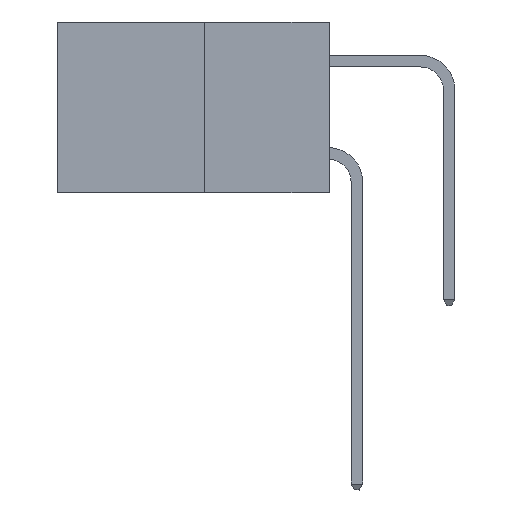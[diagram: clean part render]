
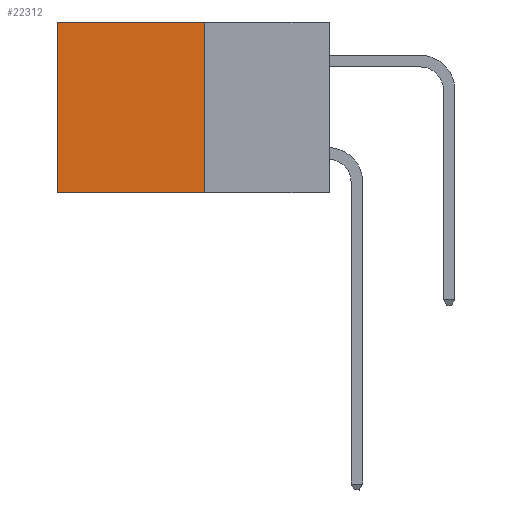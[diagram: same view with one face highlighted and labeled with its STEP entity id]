
A CAD part, left-side view. The second image highlights one B-rep face of the part: STEP entity #22312.
In plain terms, the highlighted planar face has unit normal (-1, 0, 0).
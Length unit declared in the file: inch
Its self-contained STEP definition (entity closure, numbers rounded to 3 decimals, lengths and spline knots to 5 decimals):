
#1403 = VECTOR ( 'NONE', #1879, 39.37008 ) ;
#1879 = DIRECTION ( 'NONE',  ( 0., 0., -1. ) ) ;
#2304 = CARTESIAN_POINT ( 'NONE',  ( 0.277, 0.59, -0.37 ) ) ;
#2451 = PLANE ( 'NONE',  #21595 ) ;
#4678 = ORIENTED_EDGE ( 'NONE', *, *, #18040, .F. ) ;
#8793 = ORIENTED_EDGE ( 'NONE', *, *, #16566, .F. ) ;
#9172 = CARTESIAN_POINT ( 'NONE',  ( 0.277, 0.27, -0.37 ) ) ;
#9615 = CARTESIAN_POINT ( 'NONE',  ( 0.277, 0.59, 0. ) ) ;
#10212 = VECTOR ( 'NONE', #12533, 39.37008 ) ;
#10831 = CARTESIAN_POINT ( 'NONE',  ( 0.277, 0.27, 0. ) ) ;
#10929 = VERTEX_POINT ( 'NONE', #10831 ) ;
#11396 = DIRECTION ( 'NONE',  ( 0., 0., -1. ) ) ;
#11612 = CARTESIAN_POINT ( 'NONE',  ( 0.277, 0.27, 0. ) ) ;
#11629 = LINE ( 'NONE', #21446, #10212 ) ;
#12533 = DIRECTION ( 'NONE',  ( 0., 1., 0. ) ) ;
#13137 = EDGE_CURVE ( 'NONE', #27296, #15445, #18124, .T. ) ;
#14676 = LINE ( 'NONE', #28496, #1403 ) ;
#15445 = VERTEX_POINT ( 'NONE', #2304 ) ;
#16566 = EDGE_CURVE ( 'NONE', #26795, #15445, #11629, .T. ) ;
#16731 = VECTOR ( 'NONE', #18975, 39.37008 ) ;
#16745 = VECTOR ( 'NONE', #20580, 39.37008 ) ;
#17876 = CARTESIAN_POINT ( 'NONE',  ( 0.277, 0.27, -0.37 ) ) ;
#18040 = EDGE_CURVE ( 'NONE', #10929, #26795, #14676, .T. ) ;
#18124 = LINE ( 'NONE', #18866, #16731 ) ;
#18289 = EDGE_CURVE ( 'NONE', #10929, #27296, #22664, .T. ) ;
#18866 = CARTESIAN_POINT ( 'NONE',  ( 0.277, 0.59, -0.37 ) ) ;
#18975 = DIRECTION ( 'NONE',  ( 0., 0., -1. ) ) ;
#20580 = DIRECTION ( 'NONE',  ( 0., 1., 0. ) ) ;
#21446 = CARTESIAN_POINT ( 'NONE',  ( 0.277, 0.27, -0.37 ) ) ;
#21567 = EDGE_LOOP ( 'NONE', ( #21814, #8793, #4678, #23461 ) ) ;
#21595 = AXIS2_PLACEMENT_3D ( 'NONE', #9172, #24748, #11396 ) ;
#21814 = ORIENTED_EDGE ( 'NONE', *, *, #13137, .T. ) ;
#22312 = ADVANCED_FACE ( 'NONE', ( #26950 ), #2451, .F. ) ;
#22664 = LINE ( 'NONE', #11612, #16745 ) ;
#23461 = ORIENTED_EDGE ( 'NONE', *, *, #18289, .T. ) ;
#24748 = DIRECTION ( 'NONE',  ( 1., 0., 0. ) ) ;
#26795 = VERTEX_POINT ( 'NONE', #17876 ) ;
#26950 = FACE_OUTER_BOUND ( 'NONE', #21567, .T. ) ;
#27296 = VERTEX_POINT ( 'NONE', #9615 ) ;
#28496 = CARTESIAN_POINT ( 'NONE',  ( 0.277, 0.27, -0.37 ) ) ;
